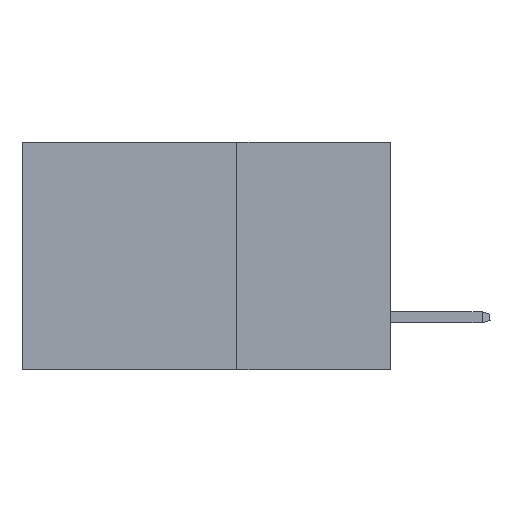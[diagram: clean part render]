
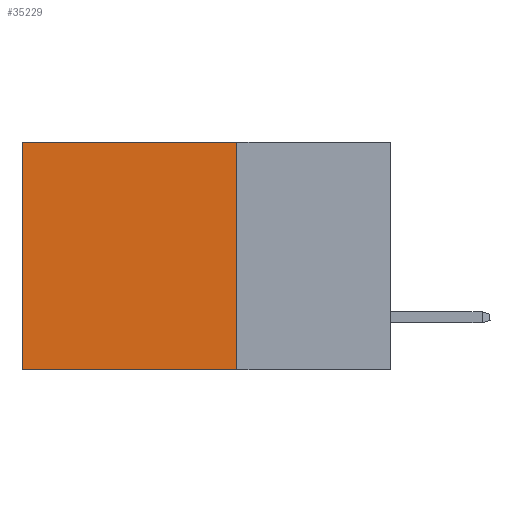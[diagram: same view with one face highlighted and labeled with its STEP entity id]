
A CAD part, left-side view. The second image highlights one B-rep face of the part: STEP entity #35229.
In plain terms, the highlighted planar face has unit normal (-1, 0, 0).
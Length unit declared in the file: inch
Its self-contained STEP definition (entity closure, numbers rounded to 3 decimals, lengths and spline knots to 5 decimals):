
#583 = EDGE_CURVE ( 'NONE', #20739, #37079, #38267, .T. ) ;
#2056 = DIRECTION ( 'NONE',  ( 0., 0., -1. ) ) ;
#2625 = CARTESIAN_POINT ( 'NONE',  ( 0.2875, 0.25, 0. ) ) ;
#2837 = ORIENTED_EDGE ( 'NONE', *, *, #35725, .T. ) ;
#3315 = ORIENTED_EDGE ( 'NONE', *, *, #4737, .F. ) ;
#4737 = EDGE_CURVE ( 'NONE', #39284, #37079, #35653, .T. ) ;
#6920 = CARTESIAN_POINT ( 'NONE',  ( 0.2875, 0.25, -0.37 ) ) ;
#7365 = DIRECTION ( 'NONE',  ( 0., 0., -1. ) ) ;
#8408 = CARTESIAN_POINT ( 'NONE',  ( 0.2875, 0.6, 0. ) ) ;
#9586 = DIRECTION ( 'NONE',  ( 0., 1., 0. ) ) ;
#12253 = CARTESIAN_POINT ( 'NONE',  ( 0.2875, 0.25, -0.37 ) ) ;
#12791 = FACE_OUTER_BOUND ( 'NONE', #45500, .T. ) ;
#14622 = VERTEX_POINT ( 'NONE', #30323 ) ;
#15496 = VECTOR ( 'NONE', #2056, 39.37008 ) ;
#16418 = VECTOR ( 'NONE', #9586, 39.37008 ) ;
#17853 = VECTOR ( 'NONE', #7365, 39.37008 ) ;
#20739 = VERTEX_POINT ( 'NONE', #8408 ) ;
#23419 = AXIS2_PLACEMENT_3D ( 'NONE', #33944, #41639, #38097 ) ;
#26962 = LINE ( 'NONE', #2625, #15496 ) ;
#28726 = CARTESIAN_POINT ( 'NONE',  ( 0.2875, 0.6, -0.37 ) ) ;
#30255 = PLANE ( 'NONE',  #23419 ) ;
#30323 = CARTESIAN_POINT ( 'NONE',  ( 0.2875, 0.25, 0. ) ) ;
#30799 = EDGE_CURVE ( 'NONE', #14622, #39284, #26962, .T. ) ;
#33944 = CARTESIAN_POINT ( 'NONE',  ( 0.2875, 0.25, 0. ) ) ;
#35229 = ADVANCED_FACE ( 'NONE', ( #12791 ), #30255, .F. ) ;
#35653 = LINE ( 'NONE', #12253, #16418 ) ;
#35725 = EDGE_CURVE ( 'NONE', #14622, #20739, #49482, .T. ) ;
#37079 = VERTEX_POINT ( 'NONE', #28726 ) ;
#38097 = DIRECTION ( 'NONE',  ( 0., 0., -1. ) ) ;
#38267 = LINE ( 'NONE', #41362, #17853 ) ;
#39284 = VERTEX_POINT ( 'NONE', #6920 ) ;
#39761 = ORIENTED_EDGE ( 'NONE', *, *, #30799, .F. ) ;
#40506 = DIRECTION ( 'NONE',  ( 0., 1., 0. ) ) ;
#41362 = CARTESIAN_POINT ( 'NONE',  ( 0.2875, 0.6, 0. ) ) ;
#41639 = DIRECTION ( 'NONE',  ( 1., 0., 0. ) ) ;
#43597 = CARTESIAN_POINT ( 'NONE',  ( 0.2875, 0.25, 0. ) ) ;
#45500 = EDGE_LOOP ( 'NONE', ( #48136, #3315, #39761, #2837 ) ) ;
#48136 = ORIENTED_EDGE ( 'NONE', *, *, #583, .T. ) ;
#48223 = VECTOR ( 'NONE', #40506, 39.37008 ) ;
#49482 = LINE ( 'NONE', #43597, #48223 ) ;
